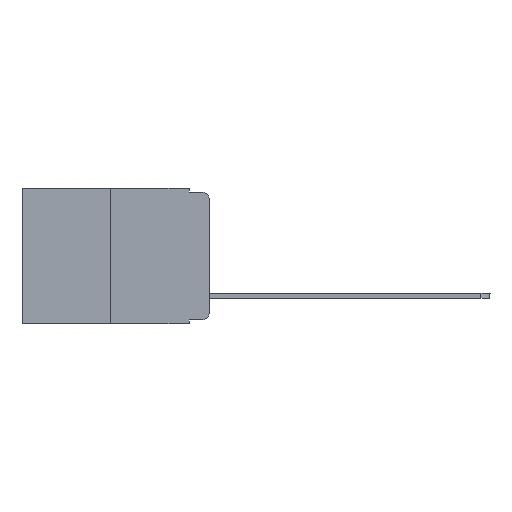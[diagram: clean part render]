
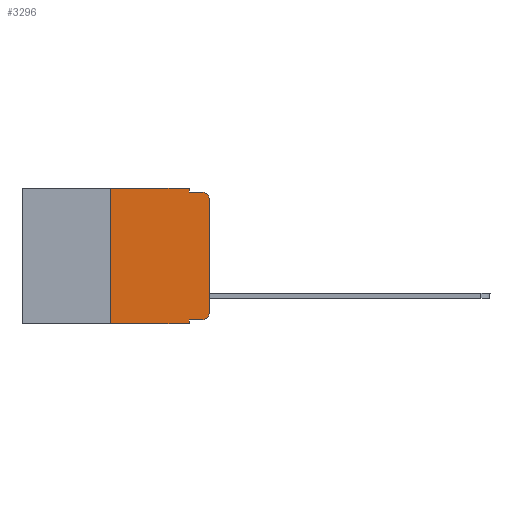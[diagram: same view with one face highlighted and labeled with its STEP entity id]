
A CAD part, left-side view. The second image highlights one B-rep face of the part: STEP entity #3296.
In plain terms, the highlighted planar face has unit normal (-1, 0, 0).
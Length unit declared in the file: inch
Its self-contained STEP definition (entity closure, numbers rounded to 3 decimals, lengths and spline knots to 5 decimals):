
#109 = EDGE_CURVE ( 'NONE', #2255, #9009, #8169, .T. ) ;
#265 = CIRCLE ( 'NONE', #942, 0.02 ) ;
#435 = ORIENTED_EDGE ( 'NONE', *, *, #5164, .F. ) ;
#503 = EDGE_CURVE ( 'NONE', #4866, #6377, #2218, .T. ) ;
#608 = DIRECTION ( 'NONE',  ( 0., 0., 1. ) ) ;
#634 = DIRECTION ( 'NONE',  ( 0., -1., 0. ) ) ;
#796 = DIRECTION ( 'NONE',  ( 0., 0., -1. ) ) ;
#942 = AXIS2_PLACEMENT_3D ( 'NONE', #1948, #11290, #11454 ) ;
#1279 = ORIENTED_EDGE ( 'NONE', *, *, #11781, .F. ) ;
#1373 = ORIENTED_EDGE ( 'NONE', *, *, #9773, .T. ) ;
#1502 = DIRECTION ( 'NONE',  ( 0., 0., -1. ) ) ;
#1771 = VERTEX_POINT ( 'NONE', #13523 ) ;
#1860 = DIRECTION ( 'NONE',  ( 0., 0., -1. ) ) ;
#1948 = CARTESIAN_POINT ( 'NONE',  ( 0., 0.02, -0.03 ) ) ;
#2218 = LINE ( 'NONE', #3627, #3494 ) ;
#2255 = VERTEX_POINT ( 'NONE', #14013 ) ;
#2590 = LINE ( 'NONE', #13695, #7608 ) ;
#2953 = VERTEX_POINT ( 'NONE', #4153 ) ;
#3296 = ADVANCED_FACE ( 'NONE', ( #8338 ), #9817, .F. ) ;
#3494 = VECTOR ( 'NONE', #9820, 39.37008 ) ;
#3627 = CARTESIAN_POINT ( 'NONE',  ( 0., 0.473, 0. ) ) ;
#3712 = DIRECTION ( 'NONE',  ( 1., 0., 0. ) ) ;
#3720 = DIRECTION ( 'NONE',  ( 0., -1., 0. ) ) ;
#3902 = DIRECTION ( 'NONE',  ( -1., 0., 0. ) ) ;
#4153 = CARTESIAN_POINT ( 'NONE',  ( 0., 0.051, -0.343 ) ) ;
#4299 = VERTEX_POINT ( 'NONE', #9066 ) ;
#4309 = VERTEX_POINT ( 'NONE', #11243 ) ;
#4537 = VECTOR ( 'NONE', #796, 39.37008 ) ;
#4749 = LINE ( 'NONE', #12437, #13692 ) ;
#4821 = AXIS2_PLACEMENT_3D ( 'NONE', #7498, #3712, #1502 ) ;
#4866 = VERTEX_POINT ( 'NONE', #6514 ) ;
#5029 = ORIENTED_EDGE ( 'NONE', *, *, #9458, .T. ) ;
#5101 = EDGE_CURVE ( 'NONE', #1771, #2953, #8827, .T. ) ;
#5154 = ORIENTED_EDGE ( 'NONE', *, *, #5101, .T. ) ;
#5164 = EDGE_CURVE ( 'NONE', #4299, #14420, #11636, .T. ) ;
#6097 = VECTOR ( 'NONE', #9586, 39.37008 ) ;
#6350 = CARTESIAN_POINT ( 'NONE',  ( 0., 0.051, 0. ) ) ;
#6377 = VERTEX_POINT ( 'NONE', #6350 ) ;
#6379 = VECTOR ( 'NONE', #3720, 39.37008 ) ;
#6453 = CARTESIAN_POINT ( 'NONE',  ( 0., 0.051, -0.01 ) ) ;
#6514 = CARTESIAN_POINT ( 'NONE',  ( 0., 0.25, 0. ) ) ;
#6528 = DIRECTION ( 'NONE',  ( 0., -1., 0. ) ) ;
#6992 = AXIS2_PLACEMENT_3D ( 'NONE', #11039, #3902, #13638 ) ;
#7369 = VERTEX_POINT ( 'NONE', #10201 ) ;
#7498 = CARTESIAN_POINT ( 'NONE',  ( 0., 0.473, 0. ) ) ;
#7608 = VECTOR ( 'NONE', #1860, 39.37008 ) ;
#8169 = LINE ( 'NONE', #11294, #13739 ) ;
#8338 = FACE_OUTER_BOUND ( 'NONE', #8566, .T. ) ;
#8566 = EDGE_LOOP ( 'NONE', ( #8627, #5029, #435, #9920, #14690, #1279, #5154, #9081, #9150, #1373 ) ) ;
#8627 = ORIENTED_EDGE ( 'NONE', *, *, #14962, .T. ) ;
#8827 = LINE ( 'NONE', #10914, #6379 ) ;
#8884 = CARTESIAN_POINT ( 'NONE',  ( 0., 0.02, -0.333 ) ) ;
#9009 = VERTEX_POINT ( 'NONE', #8884 ) ;
#9057 = EDGE_CURVE ( 'NONE', #2255, #2953, #11436, .T. ) ;
#9066 = CARTESIAN_POINT ( 'NONE',  ( 0., 0.051, -0.01 ) ) ;
#9081 = ORIENTED_EDGE ( 'NONE', *, *, #9057, .F. ) ;
#9150 = ORIENTED_EDGE ( 'NONE', *, *, #109, .T. ) ;
#9458 = EDGE_CURVE ( 'NONE', #7369, #14420, #265, .T. ) ;
#9586 = DIRECTION ( 'NONE',  ( 0., 0., 1. ) ) ;
#9670 = LINE ( 'NONE', #14304, #6097 ) ;
#9773 = EDGE_CURVE ( 'NONE', #9009, #4309, #11979, .T. ) ;
#9817 = PLANE ( 'NONE',  #4821 ) ;
#9820 = DIRECTION ( 'NONE',  ( 0., -1., 0. ) ) ;
#9920 = ORIENTED_EDGE ( 'NONE', *, *, #11424, .F. ) ;
#10201 = CARTESIAN_POINT ( 'NONE',  ( 0., 0., -0.03 ) ) ;
#10879 = VECTOR ( 'NONE', #634, 39.37008 ) ;
#10914 = CARTESIAN_POINT ( 'NONE',  ( 0., 0.473, -0.343 ) ) ;
#11039 = CARTESIAN_POINT ( 'NONE',  ( 0., 0.02, -0.313 ) ) ;
#11243 = CARTESIAN_POINT ( 'NONE',  ( 0., 0., -0.313 ) ) ;
#11290 = DIRECTION ( 'NONE',  ( -1., 0., 0. ) ) ;
#11294 = CARTESIAN_POINT ( 'NONE',  ( 0., 0.051, -0.333 ) ) ;
#11424 = EDGE_CURVE ( 'NONE', #6377, #4299, #2590, .T. ) ;
#11436 = LINE ( 'NONE', #13813, #4537 ) ;
#11454 = DIRECTION ( 'NONE',  ( 0., 0., -1. ) ) ;
#11636 = LINE ( 'NONE', #6453, #10879 ) ;
#11781 = EDGE_CURVE ( 'NONE', #1771, #4866, #9670, .T. ) ;
#11979 = CIRCLE ( 'NONE', #6992, 0.02 ) ;
#12437 = CARTESIAN_POINT ( 'NONE',  ( 0., 0., 0. ) ) ;
#13523 = CARTESIAN_POINT ( 'NONE',  ( 0., 0.25, -0.343 ) ) ;
#13638 = DIRECTION ( 'NONE',  ( 0., 0., -1. ) ) ;
#13692 = VECTOR ( 'NONE', #608, 39.37008 ) ;
#13695 = CARTESIAN_POINT ( 'NONE',  ( 0., 0.051, 0. ) ) ;
#13739 = VECTOR ( 'NONE', #6528, 39.37008 ) ;
#13813 = CARTESIAN_POINT ( 'NONE',  ( 0., 0.051, 0. ) ) ;
#14013 = CARTESIAN_POINT ( 'NONE',  ( 0., 0.051, -0.333 ) ) ;
#14304 = CARTESIAN_POINT ( 'NONE',  ( 0., 0.25, 0. ) ) ;
#14420 = VERTEX_POINT ( 'NONE', #14989 ) ;
#14690 = ORIENTED_EDGE ( 'NONE', *, *, #503, .F. ) ;
#14962 = EDGE_CURVE ( 'NONE', #4309, #7369, #4749, .T. ) ;
#14989 = CARTESIAN_POINT ( 'NONE',  ( 0., 0.02, -0.01 ) ) ;
